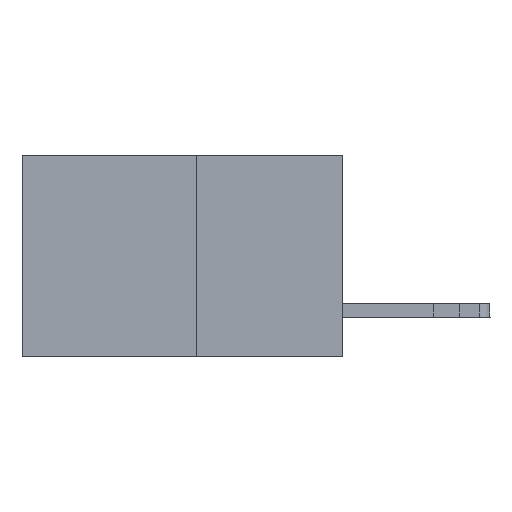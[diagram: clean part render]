
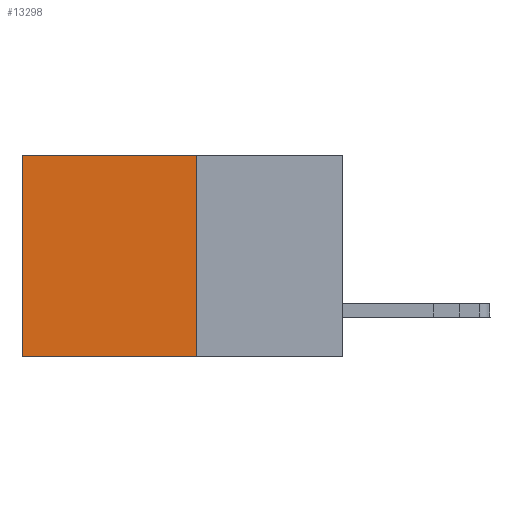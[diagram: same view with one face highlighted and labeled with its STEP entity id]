
A CAD part, left-side view. The second image highlights one B-rep face of the part: STEP entity #13298.
In plain terms, the highlighted planar face has unit normal (-1, 0, 0).
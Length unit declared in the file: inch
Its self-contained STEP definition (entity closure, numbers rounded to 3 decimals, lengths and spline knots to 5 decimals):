
#173 = FACE_OUTER_BOUND ( 'NONE', #10637, .T. ) ;
#413 = CARTESIAN_POINT ( 'NONE',  ( 0.277, 0.27, 0. ) ) ;
#500 = LINE ( 'NONE', #7342, #11330 ) ;
#528 = CARTESIAN_POINT ( 'NONE',  ( 0.277, 0.27, -0.37 ) ) ;
#1063 = VECTOR ( 'NONE', #10487, 39.37008 ) ;
#1155 = ORIENTED_EDGE ( 'NONE', *, *, #2172, .F. ) ;
#1409 = CARTESIAN_POINT ( 'NONE',  ( 0.277, 0.27, -0.37 ) ) ;
#1548 = EDGE_CURVE ( 'NONE', #2662, #1819, #500, .T. ) ;
#1819 = VERTEX_POINT ( 'NONE', #10175 ) ;
#1971 = DIRECTION ( 'NONE',  ( 0., 0., -1. ) ) ;
#2000 = AXIS2_PLACEMENT_3D ( 'NONE', #4324, #9809, #1971 ) ;
#2172 = EDGE_CURVE ( 'NONE', #2662, #5884, #8806, .T. ) ;
#2662 = VERTEX_POINT ( 'NONE', #413 ) ;
#2709 = ORIENTED_EDGE ( 'NONE', *, *, #1548, .T. ) ;
#2823 = CARTESIAN_POINT ( 'NONE',  ( 0.277, 0.59, -0.37 ) ) ;
#2945 = VECTOR ( 'NONE', #9296, 39.37008 ) ;
#3485 = CARTESIAN_POINT ( 'NONE',  ( 0.277, 0.59, -0.37 ) ) ;
#4174 = VERTEX_POINT ( 'NONE', #2823 ) ;
#4324 = CARTESIAN_POINT ( 'NONE',  ( 0.277, 0.27, -0.37 ) ) ;
#5424 = CARTESIAN_POINT ( 'NONE',  ( 0.277, 0.27, -0.37 ) ) ;
#5884 = VERTEX_POINT ( 'NONE', #1409 ) ;
#5926 = DIRECTION ( 'NONE',  ( 0., 0., -1. ) ) ;
#7342 = CARTESIAN_POINT ( 'NONE',  ( 0.277, 0.27, 0. ) ) ;
#7535 = LINE ( 'NONE', #3485, #1063 ) ;
#7858 = VECTOR ( 'NONE', #5926, 39.37008 ) ;
#8806 = LINE ( 'NONE', #528, #7858 ) ;
#9296 = DIRECTION ( 'NONE',  ( 0., 1., 0. ) ) ;
#9352 = EDGE_CURVE ( 'NONE', #5884, #4174, #13516, .T. ) ;
#9809 = DIRECTION ( 'NONE',  ( 1., 0., 0. ) ) ;
#10034 = DIRECTION ( 'NONE',  ( 0., 1., 0. ) ) ;
#10175 = CARTESIAN_POINT ( 'NONE',  ( 0.277, 0.59, 0. ) ) ;
#10487 = DIRECTION ( 'NONE',  ( 0., 0., -1. ) ) ;
#10637 = EDGE_LOOP ( 'NONE', ( #15084, #16994, #1155, #2709 ) ) ;
#11175 = EDGE_CURVE ( 'NONE', #1819, #4174, #7535, .T. ) ;
#11330 = VECTOR ( 'NONE', #10034, 39.37008 ) ;
#13298 = ADVANCED_FACE ( 'NONE', ( #173 ), #16636, .F. ) ;
#13516 = LINE ( 'NONE', #5424, #2945 ) ;
#15084 = ORIENTED_EDGE ( 'NONE', *, *, #11175, .T. ) ;
#16636 = PLANE ( 'NONE',  #2000 ) ;
#16994 = ORIENTED_EDGE ( 'NONE', *, *, #9352, .F. ) ;
